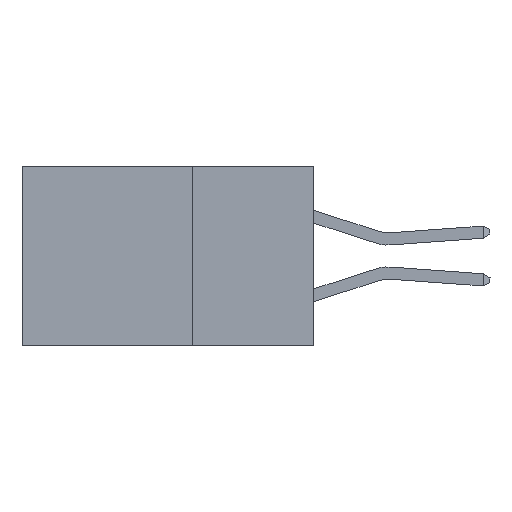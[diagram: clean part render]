
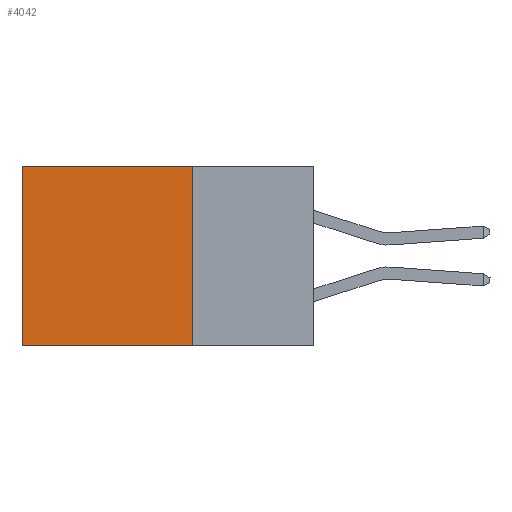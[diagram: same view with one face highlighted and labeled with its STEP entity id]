
A CAD part, left-side view. The second image highlights one B-rep face of the part: STEP entity #4042.
In plain terms, the highlighted planar face has unit normal (-1, 0, 0).
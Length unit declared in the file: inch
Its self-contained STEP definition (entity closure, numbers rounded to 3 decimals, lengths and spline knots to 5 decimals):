
#748 = EDGE_CURVE ( 'NONE', #10812, #15999, #20506, .T. ) ;
#1596 = LINE ( 'NONE', #3986, #5419 ) ;
#1777 = EDGE_LOOP ( 'NONE', ( #15446, #12675, #7936, #14316 ) ) ;
#2192 = CARTESIAN_POINT ( 'NONE',  ( 0.2875, 0.25, 0. ) ) ;
#2369 = CARTESIAN_POINT ( 'NONE',  ( 0.2875, 0.25, -0.37 ) ) ;
#3909 = CARTESIAN_POINT ( 'NONE',  ( 0.2875, 0.25, -0.37 ) ) ;
#3986 = CARTESIAN_POINT ( 'NONE',  ( 0.2875, 0.25, 0. ) ) ;
#4042 = ADVANCED_FACE ( 'NONE', ( #14426 ), #11981, .F. ) ;
#5419 = VECTOR ( 'NONE', #5611, 39.37008 ) ;
#5555 = DIRECTION ( 'NONE',  ( 1., 0., 0. ) ) ;
#5611 = DIRECTION ( 'NONE',  ( 0., 0., -1. ) ) ;
#6835 = VECTOR ( 'NONE', #15447, 39.37008 ) ;
#6931 = AXIS2_PLACEMENT_3D ( 'NONE', #2192, #5555, #16737 ) ;
#7239 = LINE ( 'NONE', #9312, #7757 ) ;
#7757 = VECTOR ( 'NONE', #15713, 39.37008 ) ;
#7936 = ORIENTED_EDGE ( 'NONE', *, *, #19863, .F. ) ;
#8062 = CARTESIAN_POINT ( 'NONE',  ( 0.2875, 0.6, 0. ) ) ;
#8162 = CARTESIAN_POINT ( 'NONE',  ( 0.2875, 0.25, 0. ) ) ;
#9312 = CARTESIAN_POINT ( 'NONE',  ( 0.2875, 0.6, 0. ) ) ;
#10812 = VERTEX_POINT ( 'NONE', #8162 ) ;
#11107 = CARTESIAN_POINT ( 'NONE',  ( 0.2875, 0.25, 0. ) ) ;
#11981 = PLANE ( 'NONE',  #6931 ) ;
#12675 = ORIENTED_EDGE ( 'NONE', *, *, #20688, .F. ) ;
#14231 = VERTEX_POINT ( 'NONE', #2369 ) ;
#14316 = ORIENTED_EDGE ( 'NONE', *, *, #748, .T. ) ;
#14426 = FACE_OUTER_BOUND ( 'NONE', #1777, .T. ) ;
#15446 = ORIENTED_EDGE ( 'NONE', *, *, #18043, .T. ) ;
#15447 = DIRECTION ( 'NONE',  ( 0., 1., 0. ) ) ;
#15558 = VECTOR ( 'NONE', #19889, 39.37008 ) ;
#15668 = VERTEX_POINT ( 'NONE', #19746 ) ;
#15713 = DIRECTION ( 'NONE',  ( 0., 0., -1. ) ) ;
#15999 = VERTEX_POINT ( 'NONE', #8062 ) ;
#16737 = DIRECTION ( 'NONE',  ( 0., 0., -1. ) ) ;
#18043 = EDGE_CURVE ( 'NONE', #15999, #15668, #7239, .T. ) ;
#19721 = LINE ( 'NONE', #3909, #15558 ) ;
#19746 = CARTESIAN_POINT ( 'NONE',  ( 0.2875, 0.6, -0.37 ) ) ;
#19863 = EDGE_CURVE ( 'NONE', #10812, #14231, #1596, .T. ) ;
#19889 = DIRECTION ( 'NONE',  ( 0., 1., 0. ) ) ;
#20506 = LINE ( 'NONE', #11107, #6835 ) ;
#20688 = EDGE_CURVE ( 'NONE', #14231, #15668, #19721, .T. ) ;
